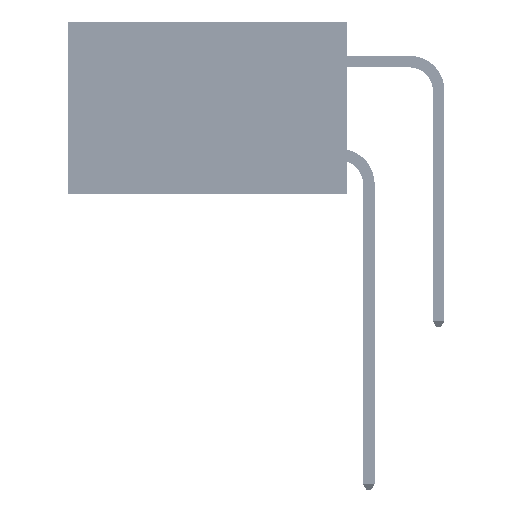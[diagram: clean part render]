
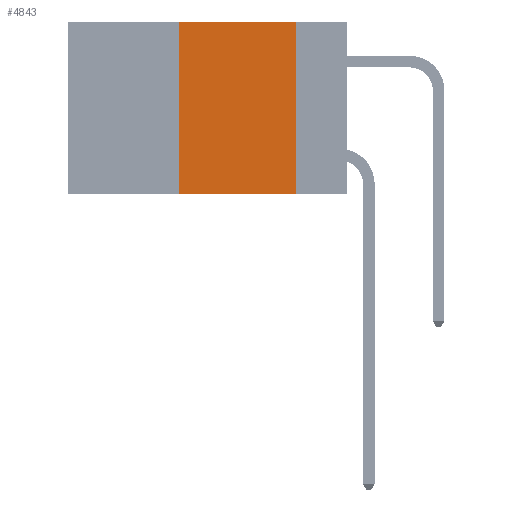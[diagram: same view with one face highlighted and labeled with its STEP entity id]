
A CAD part, left-side view. The second image highlights one B-rep face of the part: STEP entity #4843.
In plain terms, the highlighted planar face has unit normal (-1, 0, 0).
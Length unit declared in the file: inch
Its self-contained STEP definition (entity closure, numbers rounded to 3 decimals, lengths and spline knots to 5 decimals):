
#3688 = EDGE_CURVE ( 'NONE', #22321, #36110, #23408, .T. ) ;
#4843 = ADVANCED_FACE ( 'NONE', ( #26514 ), #50826, .F. ) ;
#4927 = ORIENTED_EDGE ( 'NONE', *, *, #42482, .F. ) ;
#9892 = CARTESIAN_POINT ( 'NONE',  ( 0., 0.36, 0. ) ) ;
#10155 = LINE ( 'NONE', #9892, #43455 ) ;
#10814 = CARTESIAN_POINT ( 'NONE',  ( 0., 0.11, -0.37 ) ) ;
#11072 = DIRECTION ( 'NONE',  ( 0., -1., 0. ) ) ;
#11717 = ORIENTED_EDGE ( 'NONE', *, *, #3688, .T. ) ;
#11956 = CARTESIAN_POINT ( 'NONE',  ( 0., 0.11, 0. ) ) ;
#14581 = LINE ( 'NONE', #48744, #47053 ) ;
#15962 = VERTEX_POINT ( 'NONE', #46788 ) ;
#18619 = LINE ( 'NONE', #42950, #50176 ) ;
#21568 = VERTEX_POINT ( 'NONE', #11956 ) ;
#22321 = VERTEX_POINT ( 'NONE', #29276 ) ;
#23408 = LINE ( 'NONE', #40869, #26024 ) ;
#26024 = VECTOR ( 'NONE', #11072, 39.37008 ) ;
#26514 = FACE_OUTER_BOUND ( 'NONE', #36973, .T. ) ;
#29276 = CARTESIAN_POINT ( 'NONE',  ( 0., 0.36, -0.37 ) ) ;
#30043 = EDGE_CURVE ( 'NONE', #22321, #15962, #10155, .T. ) ;
#30434 = ORIENTED_EDGE ( 'NONE', *, *, #50982, .F. ) ;
#34179 = DIRECTION ( 'NONE',  ( 1., 0., 0. ) ) ;
#35850 = ORIENTED_EDGE ( 'NONE', *, *, #30043, .F. ) ;
#36110 = VERTEX_POINT ( 'NONE', #10814 ) ;
#36854 = AXIS2_PLACEMENT_3D ( 'NONE', #51374, #34179, #50563 ) ;
#36973 = EDGE_LOOP ( 'NONE', ( #30434, #4927, #35850, #11717 ) ) ;
#38600 = DIRECTION ( 'NONE',  ( 0., 0., 1. ) ) ;
#40869 = CARTESIAN_POINT ( 'NONE',  ( 0., 0.6, -0.37 ) ) ;
#42482 = EDGE_CURVE ( 'NONE', #15962, #21568, #18619, .T. ) ;
#42950 = CARTESIAN_POINT ( 'NONE',  ( 0., 0.6, 0. ) ) ;
#43455 = VECTOR ( 'NONE', #38600, 39.37008 ) ;
#43769 = DIRECTION ( 'NONE',  ( 0., -1., 0. ) ) ;
#43845 = DIRECTION ( 'NONE',  ( 0., 0., -1. ) ) ;
#46788 = CARTESIAN_POINT ( 'NONE',  ( 0., 0.36, 0. ) ) ;
#47053 = VECTOR ( 'NONE', #43845, 39.37008 ) ;
#48744 = CARTESIAN_POINT ( 'NONE',  ( 0., 0.11, 0. ) ) ;
#50176 = VECTOR ( 'NONE', #43769, 39.37008 ) ;
#50563 = DIRECTION ( 'NONE',  ( 0., 0., -1. ) ) ;
#50826 = PLANE ( 'NONE',  #36854 ) ;
#50982 = EDGE_CURVE ( 'NONE', #21568, #36110, #14581, .T. ) ;
#51374 = CARTESIAN_POINT ( 'NONE',  ( 0., 0.6, 0. ) ) ;
